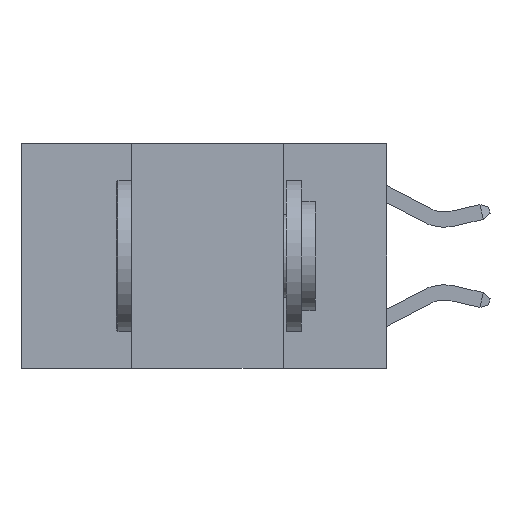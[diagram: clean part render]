
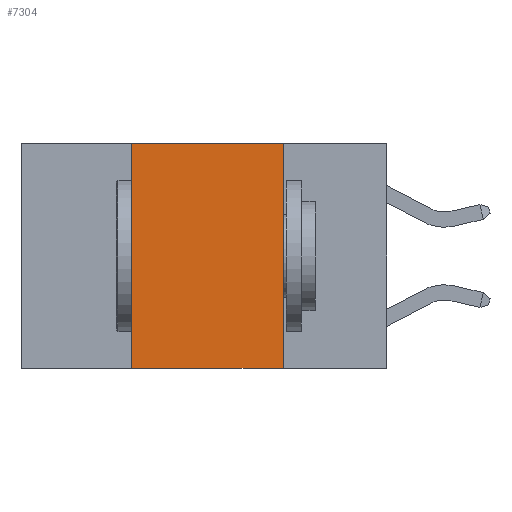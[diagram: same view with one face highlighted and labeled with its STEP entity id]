
A CAD part, left-side view. The second image highlights one B-rep face of the part: STEP entity #7304.
In plain terms, the highlighted planar face has unit normal (-1, 0, 0).
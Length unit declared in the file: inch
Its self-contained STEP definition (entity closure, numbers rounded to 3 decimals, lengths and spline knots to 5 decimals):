
#1243 = EDGE_CURVE ( 'NONE', #7094, #3003, #22028, .T. ) ;
#1755 = EDGE_CURVE ( 'NONE', #9457, #19167, #18973, .T. ) ;
#1807 = CARTESIAN_POINT ( 'NONE',  ( 0., 0.6, 0. ) ) ;
#1942 = DIRECTION ( 'NONE',  ( 0., 0., 1. ) ) ;
#3003 = VERTEX_POINT ( 'NONE', #16831 ) ;
#5052 = ORIENTED_EDGE ( 'NONE', *, *, #1755, .F. ) ;
#5850 = FACE_OUTER_BOUND ( 'NONE', #7566, .T. ) ;
#6408 = VECTOR ( 'NONE', #1942, 39.37008 ) ;
#6681 = VECTOR ( 'NONE', #13707, 39.37008 ) ;
#7094 = VERTEX_POINT ( 'NONE', #10933 ) ;
#7230 = DIRECTION ( 'NONE',  ( 0., -1., 0. ) ) ;
#7304 = ADVANCED_FACE ( 'NONE', ( #5850 ), #9563, .F. ) ;
#7566 = EDGE_LOOP ( 'NONE', ( #10473, #20854, #5052, #14048 ) ) ;
#9457 = VERTEX_POINT ( 'NONE', #22004 ) ;
#9563 = PLANE ( 'NONE',  #14041 ) ;
#10292 = CARTESIAN_POINT ( 'NONE',  ( 0., 0.6, -0.37 ) ) ;
#10398 = LINE ( 'NONE', #10292, #21948 ) ;
#10473 = ORIENTED_EDGE ( 'NONE', *, *, #1243, .F. ) ;
#10933 = CARTESIAN_POINT ( 'NONE',  ( 0., 0.17, 0. ) ) ;
#11264 = DIRECTION ( 'NONE',  ( 1., 0., 0. ) ) ;
#12820 = CARTESIAN_POINT ( 'NONE',  ( 0., 0.42, 0. ) ) ;
#13047 = DIRECTION ( 'NONE',  ( 0., 0., -1. ) ) ;
#13707 = DIRECTION ( 'NONE',  ( 0., -1., 0. ) ) ;
#14041 = AXIS2_PLACEMENT_3D ( 'NONE', #19762, #11264, #13047 ) ;
#14048 = ORIENTED_EDGE ( 'NONE', *, *, #21751, .T. ) ;
#14574 = EDGE_CURVE ( 'NONE', #19167, #7094, #20418, .T. ) ;
#15808 = VECTOR ( 'NONE', #20117, 39.37008 ) ;
#16831 = CARTESIAN_POINT ( 'NONE',  ( 0., 0.17, -0.37 ) ) ;
#17272 = CARTESIAN_POINT ( 'NONE',  ( 0., 0.42, 0. ) ) ;
#18973 = LINE ( 'NONE', #17272, #6408 ) ;
#19167 = VERTEX_POINT ( 'NONE', #12820 ) ;
#19762 = CARTESIAN_POINT ( 'NONE',  ( 0., 0.6, 0. ) ) ;
#19916 = CARTESIAN_POINT ( 'NONE',  ( 0., 0.17, 0. ) ) ;
#20117 = DIRECTION ( 'NONE',  ( 0., 0., -1. ) ) ;
#20418 = LINE ( 'NONE', #1807, #6681 ) ;
#20854 = ORIENTED_EDGE ( 'NONE', *, *, #14574, .F. ) ;
#21751 = EDGE_CURVE ( 'NONE', #9457, #3003, #10398, .T. ) ;
#21948 = VECTOR ( 'NONE', #7230, 39.37008 ) ;
#22004 = CARTESIAN_POINT ( 'NONE',  ( 0., 0.42, -0.37 ) ) ;
#22028 = LINE ( 'NONE', #19916, #15808 ) ;
